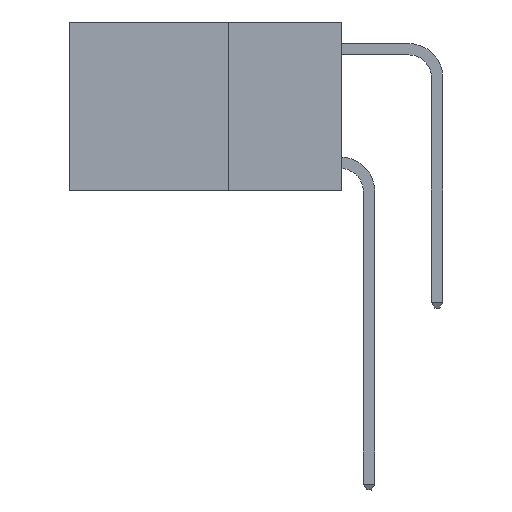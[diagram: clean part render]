
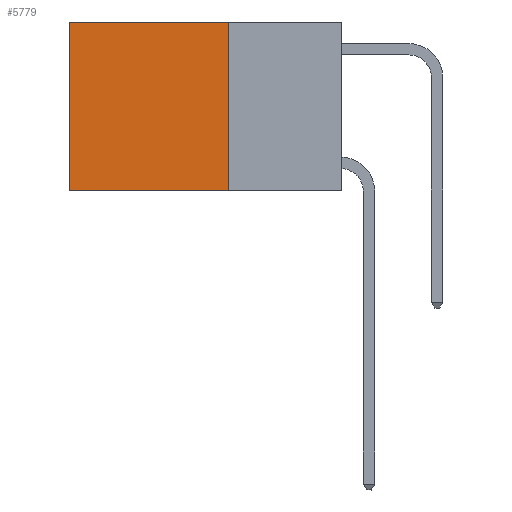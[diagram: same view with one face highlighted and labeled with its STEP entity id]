
A CAD part, left-side view. The second image highlights one B-rep face of the part: STEP entity #5779.
In plain terms, the highlighted planar face has unit normal (-1, 0, 0).
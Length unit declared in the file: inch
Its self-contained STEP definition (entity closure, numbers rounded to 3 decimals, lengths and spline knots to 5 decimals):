
#91 = FACE_OUTER_BOUND ( 'NONE', #10646, .T. ) ;
#692 = ORIENTED_EDGE ( 'NONE', *, *, #10068, .F. ) ;
#1567 = VECTOR ( 'NONE', #10656, 39.37008 ) ;
#2122 = VECTOR ( 'NONE', #6701, 39.37008 ) ;
#2454 = VECTOR ( 'NONE', #9973, 39.37008 ) ;
#2848 = LINE ( 'NONE', #6091, #2454 ) ;
#2918 = VERTEX_POINT ( 'NONE', #10613 ) ;
#3372 = CARTESIAN_POINT ( 'NONE',  ( 0.2625, 0.25, 0. ) ) ;
#5561 = LINE ( 'NONE', #15391, #2122 ) ;
#5747 = LINE ( 'NONE', #7370, #15307 ) ;
#5779 = ADVANCED_FACE ( 'NONE', ( #91 ), #14484, .F. ) ;
#6091 = CARTESIAN_POINT ( 'NONE',  ( 0.2625, 0.25, 0. ) ) ;
#6530 = EDGE_CURVE ( 'NONE', #13059, #10242, #5747, .T. ) ;
#6701 = DIRECTION ( 'NONE',  ( 0., 0., -1. ) ) ;
#7041 = DIRECTION ( 'NONE',  ( 1., 0., 0. ) ) ;
#7244 = CARTESIAN_POINT ( 'NONE',  ( 0.2625, 0.6, -0.37 ) ) ;
#7370 = CARTESIAN_POINT ( 'NONE',  ( 0.2625, 0.25, 0. ) ) ;
#7578 = ORIENTED_EDGE ( 'NONE', *, *, #6530, .F. ) ;
#9487 = ORIENTED_EDGE ( 'NONE', *, *, #15418, .T. ) ;
#9973 = DIRECTION ( 'NONE',  ( 0., 1., 0. ) ) ;
#10068 = EDGE_CURVE ( 'NONE', #10242, #13653, #10616, .T. ) ;
#10242 = VERTEX_POINT ( 'NONE', #12216 ) ;
#10602 = CARTESIAN_POINT ( 'NONE',  ( 0.2625, 0.25, -0.37 ) ) ;
#10613 = CARTESIAN_POINT ( 'NONE',  ( 0.2625, 0.6, 0. ) ) ;
#10616 = LINE ( 'NONE', #10602, #1567 ) ;
#10646 = EDGE_LOOP ( 'NONE', ( #10934, #692, #7578, #9487 ) ) ;
#10656 = DIRECTION ( 'NONE',  ( 0., 1., 0. ) ) ;
#10934 = ORIENTED_EDGE ( 'NONE', *, *, #12160, .T. ) ;
#11466 = AXIS2_PLACEMENT_3D ( 'NONE', #15628, #7041, #15686 ) ;
#12160 = EDGE_CURVE ( 'NONE', #2918, #13653, #5561, .T. ) ;
#12216 = CARTESIAN_POINT ( 'NONE',  ( 0.2625, 0.25, -0.37 ) ) ;
#13059 = VERTEX_POINT ( 'NONE', #3372 ) ;
#13596 = DIRECTION ( 'NONE',  ( 0., 0., -1. ) ) ;
#13653 = VERTEX_POINT ( 'NONE', #7244 ) ;
#14484 = PLANE ( 'NONE',  #11466 ) ;
#15307 = VECTOR ( 'NONE', #13596, 39.37008 ) ;
#15391 = CARTESIAN_POINT ( 'NONE',  ( 0.2625, 0.6, 0. ) ) ;
#15418 = EDGE_CURVE ( 'NONE', #13059, #2918, #2848, .T. ) ;
#15628 = CARTESIAN_POINT ( 'NONE',  ( 0.2625, 0.25, 0. ) ) ;
#15686 = DIRECTION ( 'NONE',  ( 0., 0., -1. ) ) ;
